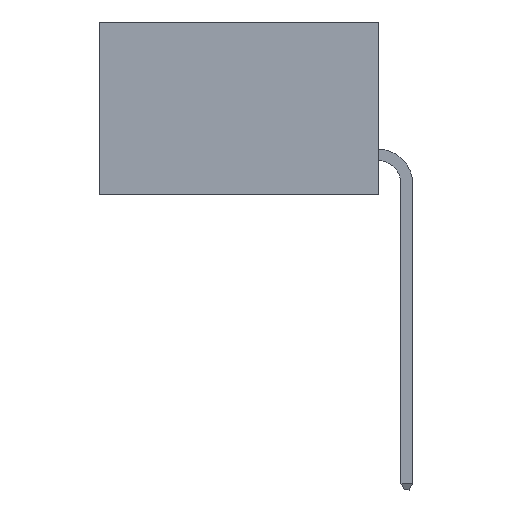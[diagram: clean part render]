
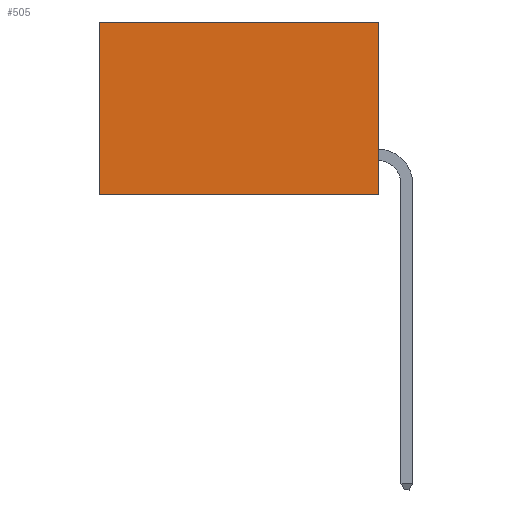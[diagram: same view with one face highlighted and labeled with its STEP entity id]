
A CAD part, left-side view. The second image highlights one B-rep face of the part: STEP entity #505.
In plain terms, the highlighted planar face has unit normal (-1, 0, 0).
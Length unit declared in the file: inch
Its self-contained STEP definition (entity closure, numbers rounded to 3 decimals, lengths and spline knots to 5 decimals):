
#121 = LINE ( 'NONE', #3078, #1322 ) ;
#311 = LINE ( 'NONE', #8768, #1398 ) ;
#505 = ADVANCED_FACE ( 'NONE', ( #3887 ), #6643, .F. ) ;
#949 = EDGE_CURVE ( 'NONE', #1854, #7549, #5340, .T. ) ;
#1205 = AXIS2_PLACEMENT_3D ( 'NONE', #9711, #4193, #4979 ) ;
#1322 = VECTOR ( 'NONE', #8688, 39.37008 ) ;
#1395 = EDGE_CURVE ( 'NONE', #2052, #7433, #2393, .T. ) ;
#1398 = VECTOR ( 'NONE', #4826, 39.37008 ) ;
#1854 = VERTEX_POINT ( 'NONE', #2673 ) ;
#2052 = VERTEX_POINT ( 'NONE', #9218 ) ;
#2393 = LINE ( 'NONE', #4915, #7924 ) ;
#2409 = ORIENTED_EDGE ( 'NONE', *, *, #3202, .T. ) ;
#2673 = CARTESIAN_POINT ( 'NONE',  ( 0.298, 0.6, 0. ) ) ;
#2884 = CARTESIAN_POINT ( 'NONE',  ( 0.298, 0., -0.37 ) ) ;
#3078 = CARTESIAN_POINT ( 'NONE',  ( 0.298, 0., -0.37 ) ) ;
#3202 = EDGE_CURVE ( 'NONE', #2052, #1854, #311, .T. ) ;
#3821 = DIRECTION ( 'NONE',  ( 0., 0., -1. ) ) ;
#3887 = FACE_OUTER_BOUND ( 'NONE', #7850, .T. ) ;
#4193 = DIRECTION ( 'NONE',  ( 1., 0., 0. ) ) ;
#4826 = DIRECTION ( 'NONE',  ( 0., 1., 0. ) ) ;
#4868 = ORIENTED_EDGE ( 'NONE', *, *, #949, .T. ) ;
#4915 = CARTESIAN_POINT ( 'NONE',  ( 0.298, 0., 0. ) ) ;
#4979 = DIRECTION ( 'NONE',  ( 0., 0., -1. ) ) ;
#5340 = LINE ( 'NONE', #9165, #5948 ) ;
#5948 = VECTOR ( 'NONE', #6693, 39.37008 ) ;
#6169 = EDGE_CURVE ( 'NONE', #7433, #7549, #121, .T. ) ;
#6643 = PLANE ( 'NONE',  #1205 ) ;
#6693 = DIRECTION ( 'NONE',  ( 0., 0., -1. ) ) ;
#7382 = ORIENTED_EDGE ( 'NONE', *, *, #6169, .F. ) ;
#7433 = VERTEX_POINT ( 'NONE', #2884 ) ;
#7549 = VERTEX_POINT ( 'NONE', #9697 ) ;
#7850 = EDGE_LOOP ( 'NONE', ( #4868, #7382, #9762, #2409 ) ) ;
#7924 = VECTOR ( 'NONE', #3821, 39.37008 ) ;
#8688 = DIRECTION ( 'NONE',  ( 0., 1., 0. ) ) ;
#8768 = CARTESIAN_POINT ( 'NONE',  ( 0.298, 0., 0. ) ) ;
#9165 = CARTESIAN_POINT ( 'NONE',  ( 0.298, 0.6, 0. ) ) ;
#9218 = CARTESIAN_POINT ( 'NONE',  ( 0.298, 0., 0. ) ) ;
#9697 = CARTESIAN_POINT ( 'NONE',  ( 0.298, 0.6, -0.37 ) ) ;
#9711 = CARTESIAN_POINT ( 'NONE',  ( 0.298, 0., 0. ) ) ;
#9762 = ORIENTED_EDGE ( 'NONE', *, *, #1395, .F. ) ;
